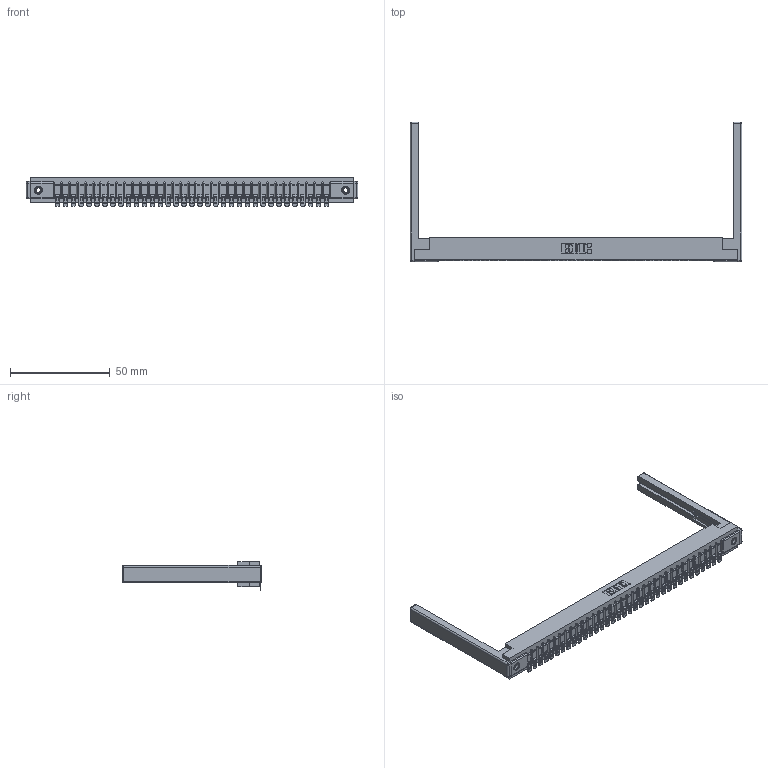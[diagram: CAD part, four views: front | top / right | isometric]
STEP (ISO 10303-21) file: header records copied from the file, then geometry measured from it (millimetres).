
FILE_DESCRIPTION (( 'STEP AP203' ), '1' );
FILE_NAME ('357-035-554-168.STEP', '2019-09-17T06:13:55', ( '' ), ( '' ), 'SwSTEP 2.0', 'SolidWorks 2016', '' );
FILE_SCHEMA (( 'CONFIG_CONTROL_DESIGN' ));
Length unit declared in the file: inch
Products named in the file (5): 345-250-001_345-250-001-102; 307-290-002_554; 357-035-554-168; 307 Part_.156 Dia Mounting Holes; 307-220-068
Assembly tree (40 placements, depth 2):
  357-035-554-168
    307 Part_.156 Dia Mounting Holes
    307-290-002_554  x35
    307-220-068  x2
    345-250-001_345-250-001-102  x2
Bounding box: 166.12 x 69.98 x 14.52 mm (x, y, z)
Volume: 22114.5 mm3; surface area: 26244.3 mm2
Topology: 40 solids, 40 shells, 3143 faces, 9568 edges, 6260 vertices
Faces by surface type: plane 1768, cylinder 1279, sphere 80, cone 12, torus 4
Entity records: 34592 total; most frequent: CARTESIAN_POINT 5799, ORIENTED_EDGE 5778, DIRECTION 5661, EDGE_CURVE 2889, LINE 2201, VECTOR 2201, VERTEX_POINT 1868, AXIS2_PLACEMENT_3D 1730
